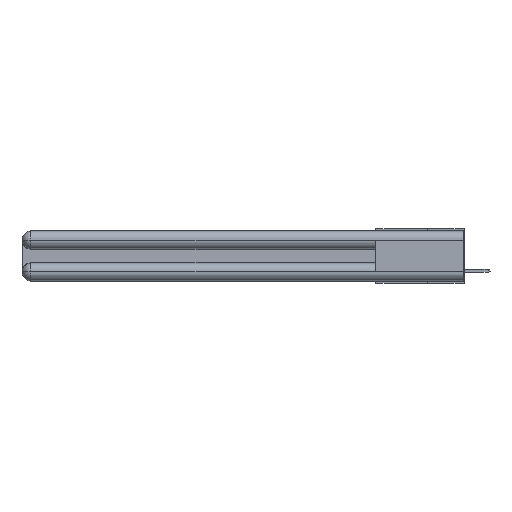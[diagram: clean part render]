
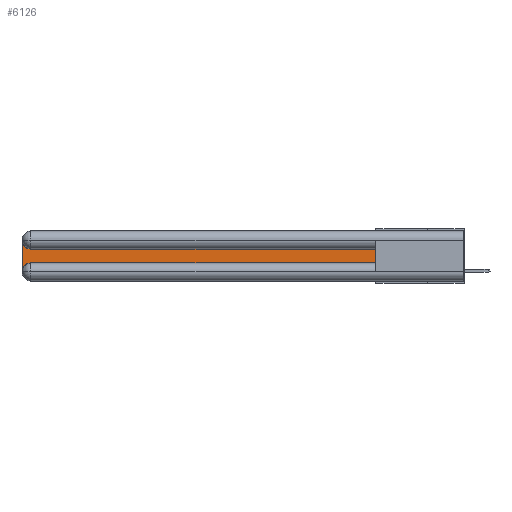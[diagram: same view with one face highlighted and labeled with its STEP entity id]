
A CAD part, left-side view. The second image highlights one B-rep face of the part: STEP entity #6126.
In plain terms, the highlighted planar face has unit normal (-1, 0, 0).
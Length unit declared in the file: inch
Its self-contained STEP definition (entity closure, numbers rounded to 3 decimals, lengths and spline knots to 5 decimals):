
#451 = VERTEX_POINT ( 'NONE', #5053 ) ;
#542 = VERTEX_POINT ( 'NONE', #28054 ) ;
#893 = EDGE_CURVE ( 'NONE', #542, #3428, #10912, .T. ) ;
#975 = ORIENTED_EDGE ( 'NONE', *, *, #893, .T. ) ;
#3087 = DIRECTION ( 'NONE',  ( 0., 0., -1. ) ) ;
#3428 = VERTEX_POINT ( 'NONE', #13949 ) ;
#4447 = DIRECTION ( 'NONE',  ( 0., -1., 0. ) ) ;
#5053 = CARTESIAN_POINT ( 'NONE',  ( 0.075, 0.6, -0.1225 ) ) ;
#6126 = ADVANCED_FACE ( 'NONE', ( #32717 ), #16973, .F. ) ;
#6188 = ORIENTED_EDGE ( 'NONE', *, *, #15432, .T. ) ;
#7590 = EDGE_LOOP ( 'NONE', ( #23738, #26863, #30044, #975, #6188, #13661 ) ) ;
#7966 = VECTOR ( 'NONE', #15007, 39.37008 ) ;
#8020 = CARTESIAN_POINT ( 'NONE',  ( 0.075, 2.94, -0.1225 ) ) ;
#8113 = DIRECTION ( 'NONE',  ( 0., 0., -1. ) ) ;
#8569 = AXIS2_PLACEMENT_3D ( 'NONE', #23734, #18498, #3087 ) ;
#9300 = DIRECTION ( 'NONE',  ( 1., 0., 0. ) ) ;
#9332 = DIRECTION ( 'NONE',  ( 1., 0., 0. ) ) ;
#9711 = CARTESIAN_POINT ( 'NONE',  ( 0.075, 0.6, -0.2175 ) ) ;
#10912 = CIRCLE ( 'NONE', #30483, 0.06 ) ;
#11192 = LINE ( 'NONE', #9711, #30120 ) ;
#11417 = VERTEX_POINT ( 'NONE', #22335 ) ;
#13000 = LINE ( 'NONE', #26469, #30740 ) ;
#13661 = ORIENTED_EDGE ( 'NONE', *, *, #16909, .T. ) ;
#13949 = CARTESIAN_POINT ( 'NONE',  ( 0.075, 2.94, -0.2175 ) ) ;
#14420 = AXIS2_PLACEMENT_3D ( 'NONE', #24700, #9300, #19676 ) ;
#14681 = VERTEX_POINT ( 'NONE', #16650 ) ;
#15007 = DIRECTION ( 'NONE',  ( 0., 1., 0. ) ) ;
#15432 = EDGE_CURVE ( 'NONE', #3428, #14681, #17786, .T. ) ;
#16650 = CARTESIAN_POINT ( 'NONE',  ( 0.075, 0.6, -0.2175 ) ) ;
#16909 = EDGE_CURVE ( 'NONE', #14681, #451, #11192, .T. ) ;
#16973 = PLANE ( 'NONE',  #14420 ) ;
#17418 = VERTEX_POINT ( 'NONE', #8020 ) ;
#17786 = LINE ( 'NONE', #32792, #28231 ) ;
#18498 = DIRECTION ( 'NONE',  ( 1., 0., 0. ) ) ;
#18523 = EDGE_CURVE ( 'NONE', #17418, #11417, #23927, .T. ) ;
#19676 = DIRECTION ( 'NONE',  ( 0., 0., -1. ) ) ;
#20119 = EDGE_CURVE ( 'NONE', #11417, #542, #13000, .T. ) ;
#22335 = CARTESIAN_POINT ( 'NONE',  ( 0.075, 3., -0.0625 ) ) ;
#23296 = LINE ( 'NONE', #30303, #7966 ) ;
#23734 = CARTESIAN_POINT ( 'NONE',  ( 0.075, 2.94, -0.0625 ) ) ;
#23738 = ORIENTED_EDGE ( 'NONE', *, *, #29211, .T. ) ;
#23927 = CIRCLE ( 'NONE', #8569, 0.06 ) ;
#24700 = CARTESIAN_POINT ( 'NONE',  ( 0.075, 3., -0.1225 ) ) ;
#24736 = CARTESIAN_POINT ( 'NONE',  ( 0.075, 2.94, -0.2775 ) ) ;
#25448 = DIRECTION ( 'NONE',  ( 0., 0., 1. ) ) ;
#26469 = CARTESIAN_POINT ( 'NONE',  ( 0.075, 3., -0.2175 ) ) ;
#26863 = ORIENTED_EDGE ( 'NONE', *, *, #18523, .T. ) ;
#27344 = DIRECTION ( 'NONE',  ( 0., 0., -1. ) ) ;
#28054 = CARTESIAN_POINT ( 'NONE',  ( 0.075, 3., -0.2775 ) ) ;
#28231 = VECTOR ( 'NONE', #4447, 39.37008 ) ;
#29211 = EDGE_CURVE ( 'NONE', #451, #17418, #23296, .T. ) ;
#30044 = ORIENTED_EDGE ( 'NONE', *, *, #20119, .T. ) ;
#30120 = VECTOR ( 'NONE', #25448, 39.37008 ) ;
#30303 = CARTESIAN_POINT ( 'NONE',  ( 0.075, 0.6, -0.1225 ) ) ;
#30483 = AXIS2_PLACEMENT_3D ( 'NONE', #24736, #9332, #27344 ) ;
#30740 = VECTOR ( 'NONE', #8113, 39.37008 ) ;
#32717 = FACE_OUTER_BOUND ( 'NONE', #7590, .T. ) ;
#32792 = CARTESIAN_POINT ( 'NONE',  ( 0.075, 0.6, -0.2175 ) ) ;
